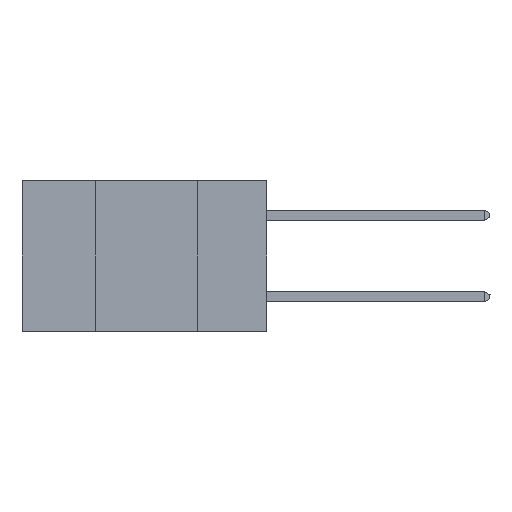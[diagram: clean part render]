
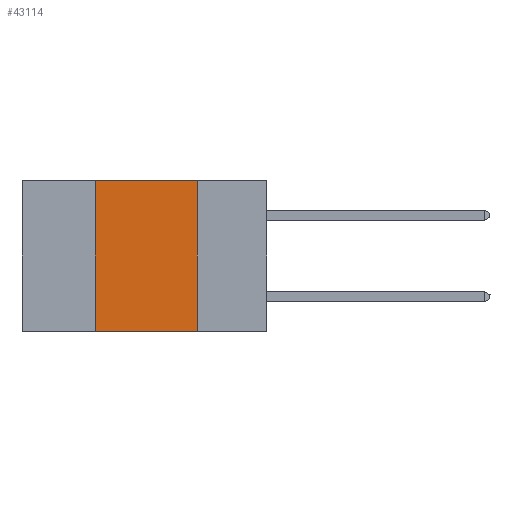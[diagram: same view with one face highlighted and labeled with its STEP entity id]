
A CAD part, left-side view. The second image highlights one B-rep face of the part: STEP entity #43114.
In plain terms, the highlighted planar face has unit normal (-1, 0, 0).
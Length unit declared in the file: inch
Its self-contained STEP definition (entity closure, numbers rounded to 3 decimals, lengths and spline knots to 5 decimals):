
#25 = CARTESIAN_POINT ( 'NONE',  ( 0., 0.17, 0. ) ) ;
#342 = VECTOR ( 'NONE', #13599, 39.37008 ) ;
#1301 = DIRECTION ( 'NONE',  ( 0., 0., -1. ) ) ;
#1514 = CARTESIAN_POINT ( 'NONE',  ( 0., 0.6, -0.37 ) ) ;
#1954 = LINE ( 'NONE', #1514, #22362 ) ;
#2169 = VECTOR ( 'NONE', #14469, 39.37008 ) ;
#2641 = ORIENTED_EDGE ( 'NONE', *, *, #43128, .T. ) ;
#3664 = VERTEX_POINT ( 'NONE', #27544 ) ;
#5104 = LINE ( 'NONE', #17815, #25156 ) ;
#5446 = VERTEX_POINT ( 'NONE', #42757 ) ;
#8209 = FACE_OUTER_BOUND ( 'NONE', #13607, .T. ) ;
#13599 = DIRECTION ( 'NONE',  ( 0., 0., -1. ) ) ;
#13607 = EDGE_LOOP ( 'NONE', ( #37875, #22485, #29906, #2641 ) ) ;
#14469 = DIRECTION ( 'NONE',  ( 0., 0., 1. ) ) ;
#15320 = DIRECTION ( 'NONE',  ( 0., -1., 0. ) ) ;
#17139 = LINE ( 'NONE', #17575, #2169 ) ;
#17575 = CARTESIAN_POINT ( 'NONE',  ( 0., 0.42, 0. ) ) ;
#17815 = CARTESIAN_POINT ( 'NONE',  ( 0., 0.6, 0. ) ) ;
#18648 = EDGE_CURVE ( 'NONE', #3664, #5446, #5104, .T. ) ;
#18726 = CARTESIAN_POINT ( 'NONE',  ( 0., 0.42, -0.37 ) ) ;
#21790 = CARTESIAN_POINT ( 'NONE',  ( 0., 0.6, 0. ) ) ;
#22362 = VECTOR ( 'NONE', #15320, 39.37008 ) ;
#22485 = ORIENTED_EDGE ( 'NONE', *, *, #18648, .F. ) ;
#23253 = VERTEX_POINT ( 'NONE', #18726 ) ;
#23651 = EDGE_CURVE ( 'NONE', #5446, #33715, #23850, .T. ) ;
#23850 = LINE ( 'NONE', #25, #342 ) ;
#25156 = VECTOR ( 'NONE', #42279, 39.37008 ) ;
#27544 = CARTESIAN_POINT ( 'NONE',  ( 0., 0.42, 0. ) ) ;
#29906 = ORIENTED_EDGE ( 'NONE', *, *, #33483, .F. ) ;
#33483 = EDGE_CURVE ( 'NONE', #23253, #3664, #17139, .T. ) ;
#33715 = VERTEX_POINT ( 'NONE', #35371 ) ;
#35371 = CARTESIAN_POINT ( 'NONE',  ( 0., 0.17, -0.37 ) ) ;
#37875 = ORIENTED_EDGE ( 'NONE', *, *, #23651, .F. ) ;
#38917 = DIRECTION ( 'NONE',  ( 1., 0., 0. ) ) ;
#39137 = PLANE ( 'NONE',  #41564 ) ;
#41564 = AXIS2_PLACEMENT_3D ( 'NONE', #21790, #38917, #1301 ) ;
#42279 = DIRECTION ( 'NONE',  ( 0., -1., 0. ) ) ;
#42757 = CARTESIAN_POINT ( 'NONE',  ( 0., 0.17, 0. ) ) ;
#43114 = ADVANCED_FACE ( 'NONE', ( #8209 ), #39137, .F. ) ;
#43128 = EDGE_CURVE ( 'NONE', #23253, #33715, #1954, .T. ) ;
